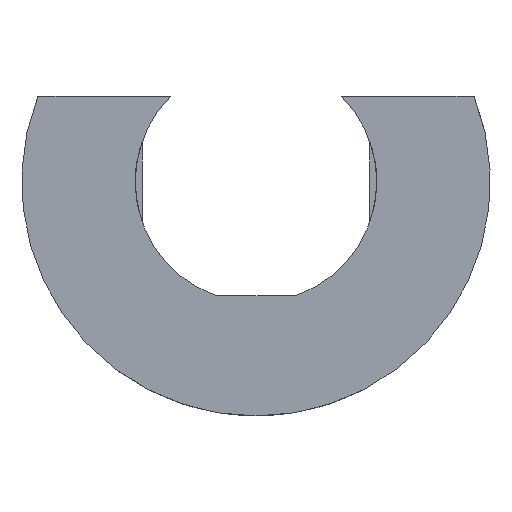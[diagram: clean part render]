
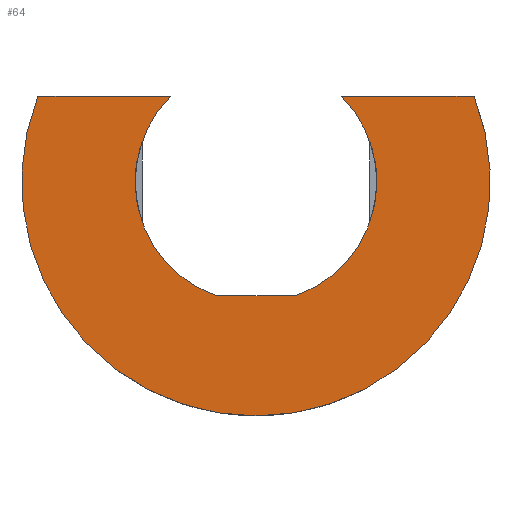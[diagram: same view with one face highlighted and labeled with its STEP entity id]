
A CAD part, front view. The second image highlights one B-rep face of the part: STEP entity #64.
In plain terms, the highlighted planar face has unit normal (0, -1, 0).
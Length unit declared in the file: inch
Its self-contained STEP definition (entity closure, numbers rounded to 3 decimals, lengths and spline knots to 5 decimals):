
#11 = EDGE_CURVE ( 'NONE', #298, #292, #324, .T. ) ;
#18 = EDGE_CURVE ( 'NONE', #277, #278, #322, .T. ) ;
#20 = EDGE_CURVE ( 'NONE', #298, #278, #58, .T. ) ;
#21 = EDGE_CURVE ( 'NONE', #292, #288, #40, .T. ) ;
#23 = EDGE_CURVE ( 'NONE', #288, #290, #47, .T. ) ;
#28 = EDGE_CURVE ( 'NONE', #277, #294, #41, .T. ) ;
#37 = EDGE_CURVE ( 'NONE', #294, #290, #412, .T. ) ;
#40 = CIRCLE ( 'NONE', #100, 1.16 ) ;
#41 = CIRCLE ( 'NONE', #95, 0.59805 ) ;
#47 = CIRCLE ( 'NONE', #113, 1.16 ) ;
#58 = CIRCLE ( 'NONE', #89, 0.59805 ) ;
#64 = ADVANCED_FACE ( 'NONE', ( #155 ), #458, .F. ) ;
#84 = VECTOR ( 'NONE', #326, 39.37008 ) ;
#89 = AXIS2_PLACEMENT_3D ( 'NONE', #315, #311, #325 ) ;
#95 = AXIS2_PLACEMENT_3D ( 'NONE', #395, #391, #378 ) ;
#100 = AXIS2_PLACEMENT_3D ( 'NONE', #313, #314, #354 ) ;
#111 = VECTOR ( 'NONE', #307, 39.37008 ) ;
#113 = AXIS2_PLACEMENT_3D ( 'NONE', #351, #343, #356 ) ;
#130 = VECTOR ( 'NONE', #414, 39.37008 ) ;
#143 = AXIS2_PLACEMENT_3D ( 'NONE', #484, #477, #459 ) ;
#155 = FACE_OUTER_BOUND ( 'NONE', #255, .T. ) ;
#209 = ORIENTED_EDGE ( 'NONE', *, *, #18, .F. ) ;
#214 = ORIENTED_EDGE ( 'NONE', *, *, #37, .T. ) ;
#216 = ORIENTED_EDGE ( 'NONE', *, *, #11, .F. ) ;
#224 = ORIENTED_EDGE ( 'NONE', *, *, #23, .F. ) ;
#229 = ORIENTED_EDGE ( 'NONE', *, *, #20, .T. ) ;
#234 = ORIENTED_EDGE ( 'NONE', *, *, #28, .T. ) ;
#255 = EDGE_LOOP ( 'NONE', ( #216, #229, #209, #234, #214, #224, #263 ) ) ;
#263 = ORIENTED_EDGE ( 'NONE', *, *, #21, .F. ) ;
#277 = VERTEX_POINT ( 'NONE', #505 ) ;
#278 = VERTEX_POINT ( 'NONE', #516 ) ;
#288 = VERTEX_POINT ( 'NONE', #499 ) ;
#290 = VERTEX_POINT ( 'NONE', #506 ) ;
#292 = VERTEX_POINT ( 'NONE', #496 ) ;
#294 = VERTEX_POINT ( 'NONE', #517 ) ;
#298 = VERTEX_POINT ( 'NONE', #500 ) ;
#307 = DIRECTION ( 'NONE',  ( 1., 0., 0. ) ) ;
#311 = DIRECTION ( 'NONE',  ( 0., 1., 0. ) ) ;
#313 = CARTESIAN_POINT ( 'NONE',  ( 0.56388, 0., -0.19685 ) ) ;
#314 = DIRECTION ( 'NONE',  ( 0., 1., 0. ) ) ;
#315 = CARTESIAN_POINT ( 'NONE',  ( 0.56388, 0., -0.19685 ) ) ;
#322 = LINE ( 'NONE', #334, #111 ) ;
#324 = LINE ( 'NONE', #327, #84 ) ;
#325 = DIRECTION ( 'NONE',  ( 0., 0., 1. ) ) ;
#326 = DIRECTION ( 'NONE',  ( 1., 0., 0. ) ) ;
#327 = CARTESIAN_POINT ( 'NONE',  ( 0., 0., 0.22676 ) ) ;
#334 = CARTESIAN_POINT ( 'NONE',  ( 0., 0., -0.76203 ) ) ;
#343 = DIRECTION ( 'NONE',  ( 0., 1., 0. ) ) ;
#351 = CARTESIAN_POINT ( 'NONE',  ( 0.56388, 0., -0.19685 ) ) ;
#354 = DIRECTION ( 'NONE',  ( 0., 0., 1. ) ) ;
#356 = DIRECTION ( 'NONE',  ( 0., 0., 1. ) ) ;
#378 = DIRECTION ( 'NONE',  ( 0., 0., 1. ) ) ;
#391 = DIRECTION ( 'NONE',  ( 0., 1., 0. ) ) ;
#395 = CARTESIAN_POINT ( 'NONE',  ( 0.56388, 0., -0.19685 ) ) ;
#412 = LINE ( 'NONE', #416, #130 ) ;
#414 = DIRECTION ( 'NONE',  ( -1., 0., 0. ) ) ;
#416 = CARTESIAN_POINT ( 'NONE',  ( 0., 0., 0.22676 ) ) ;
#458 = PLANE ( 'NONE',  #143 ) ;
#459 = DIRECTION ( 'NONE',  ( 0., 0., 1. ) ) ;
#477 = DIRECTION ( 'NONE',  ( 0., 1., 0. ) ) ;
#484 = CARTESIAN_POINT ( 'NONE',  ( 0., 0., 0. ) ) ;
#496 = CARTESIAN_POINT ( 'NONE',  ( 1.64377, 0., 0.22676 ) ) ;
#499 = CARTESIAN_POINT ( 'NONE',  ( 0.56388, 0., -1.35685 ) ) ;
#500 = CARTESIAN_POINT ( 'NONE',  ( 0.98605, 0., 0.22676 ) ) ;
#505 = CARTESIAN_POINT ( 'NONE',  ( 0.36833, 0., -0.76203 ) ) ;
#506 = CARTESIAN_POINT ( 'NONE',  ( -0.51601, 0., 0.22676 ) ) ;
#516 = CARTESIAN_POINT ( 'NONE',  ( 0.75943, 0., -0.76203 ) ) ;
#517 = CARTESIAN_POINT ( 'NONE',  ( 0.14172, 0., 0.22676 ) ) ;
